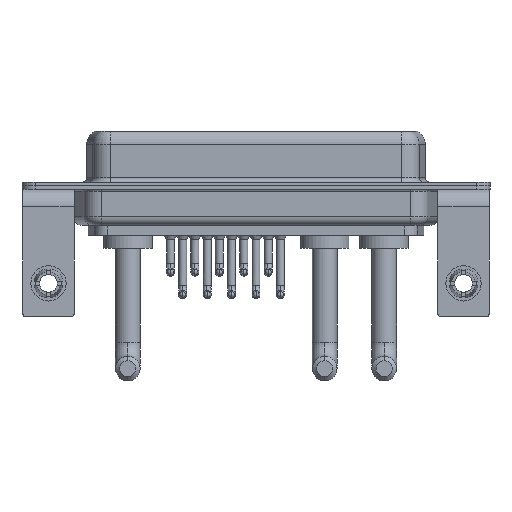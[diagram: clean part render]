
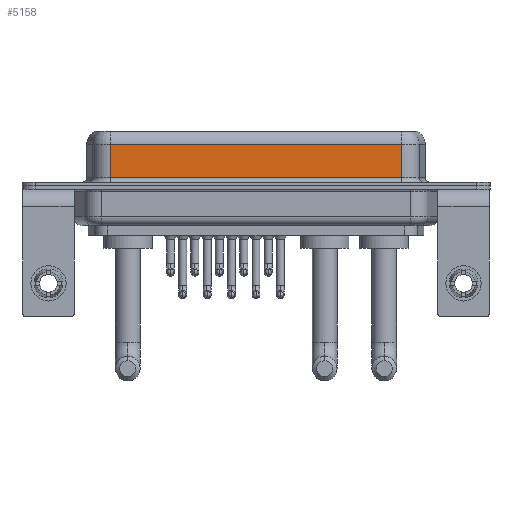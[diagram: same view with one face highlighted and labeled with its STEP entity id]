
A CAD part, front view. The second image highlights one B-rep face of the part: STEP entity #5158.
In plain terms, the highlighted planar face has unit normal (0, -1, 0).
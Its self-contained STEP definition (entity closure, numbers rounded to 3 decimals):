
#58 = CARTESIAN_POINT ( 'NONE',  ( 40.037, -3.95, 4.65 ) ) ;
#126 = DIRECTION ( 'NONE',  ( 0., 0., -1. ) ) ;
#579 = VECTOR ( 'NONE', #126, 1000. ) ;
#599 = ORIENTED_EDGE ( 'NONE', *, *, #10545, .F. ) ;
#719 = CARTESIAN_POINT ( 'NONE',  ( 40.037, -3.95, 6.4 ) ) ;
#1117 = ORIENTED_EDGE ( 'NONE', *, *, #9311, .T. ) ;
#1436 = LINE ( 'NONE', #3391, #579 ) ;
#1584 = VERTEX_POINT ( 'NONE', #18457 ) ;
#2017 = VERTEX_POINT ( 'NONE', #18435 ) ;
#2238 = VECTOR ( 'NONE', #12763, 1000. ) ;
#3391 = CARTESIAN_POINT ( 'NONE',  ( 7.013, -3.95, 6.4 ) ) ;
#3637 = CARTESIAN_POINT ( 'NONE',  ( 40.037, -3.95, 0.9 ) ) ;
#3893 = CARTESIAN_POINT ( 'NONE',  ( 40.037, -3.95, 6.4 ) ) ;
#4171 = ORIENTED_EDGE ( 'NONE', *, *, #13229, .T. ) ;
#4303 = AXIS2_PLACEMENT_3D ( 'NONE', #3893, #10500, #17232 ) ;
#5158 = ADVANCED_FACE ( 'NONE', ( #12224 ), #10608, .F. ) ;
#7428 = DIRECTION ( 'NONE',  ( 0., 0., -1. ) ) ;
#9311 = EDGE_CURVE ( 'NONE', #2017, #11402, #1436, .T. ) ;
#9437 = DIRECTION ( 'NONE',  ( 1., 0., 0. ) ) ;
#10500 = DIRECTION ( 'NONE',  ( 0., 1., 0. ) ) ;
#10545 = EDGE_CURVE ( 'NONE', #1584, #16546, #18818, .T. ) ;
#10608 = PLANE ( 'NONE',  #4303 ) ;
#11358 = ORIENTED_EDGE ( 'NONE', *, *, #17546, .T. ) ;
#11402 = VERTEX_POINT ( 'NONE', #21264 ) ;
#12224 = FACE_OUTER_BOUND ( 'NONE', #12511, .T. ) ;
#12511 = EDGE_LOOP ( 'NONE', ( #599, #11358, #1117, #4171 ) ) ;
#12763 = DIRECTION ( 'NONE',  ( -1., 0., 0. ) ) ;
#13229 = EDGE_CURVE ( 'NONE', #11402, #16546, #21032, .T. ) ;
#13877 = VECTOR ( 'NONE', #9437, 1000. ) ;
#16341 = LINE ( 'NONE', #58, #2238 ) ;
#16546 = VERTEX_POINT ( 'NONE', #3637 ) ;
#17232 = DIRECTION ( 'NONE',  ( 0., 0., 1. ) ) ;
#17546 = EDGE_CURVE ( 'NONE', #1584, #2017, #16341, .T. ) ;
#18435 = CARTESIAN_POINT ( 'NONE',  ( 7.013, -3.95, 4.65 ) ) ;
#18457 = CARTESIAN_POINT ( 'NONE',  ( 40.037, -3.95, 4.65 ) ) ;
#18818 = LINE ( 'NONE', #719, #19327 ) ;
#19327 = VECTOR ( 'NONE', #7428, 1000. ) ;
#20917 = CARTESIAN_POINT ( 'NONE',  ( 40.037, -3.95, 0.9 ) ) ;
#21032 = LINE ( 'NONE', #20917, #13877 ) ;
#21264 = CARTESIAN_POINT ( 'NONE',  ( 7.013, -3.95, 0.9 ) ) ;
